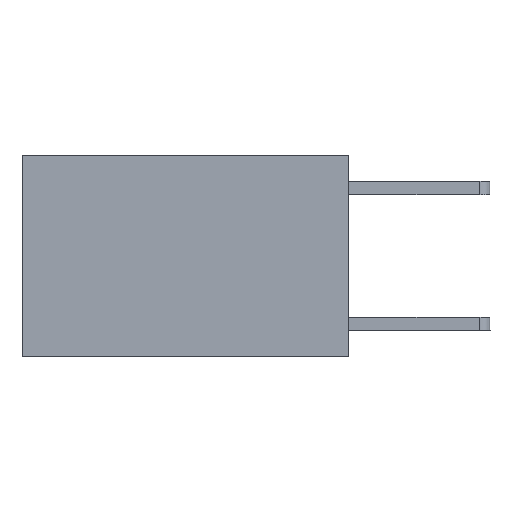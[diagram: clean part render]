
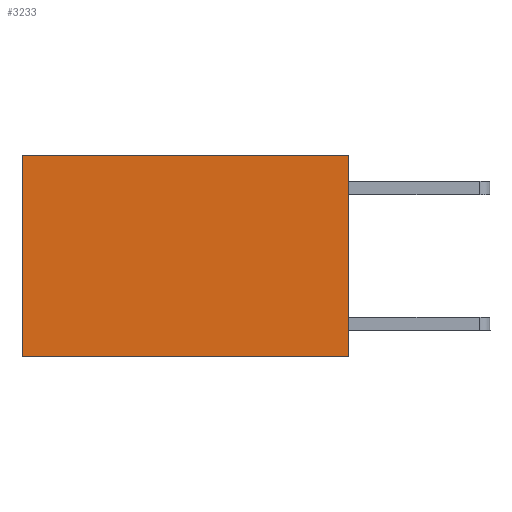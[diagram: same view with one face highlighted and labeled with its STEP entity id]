
A CAD part, left-side view. The second image highlights one B-rep face of the part: STEP entity #3233.
In plain terms, the highlighted planar face has unit normal (-1, 0, 0).
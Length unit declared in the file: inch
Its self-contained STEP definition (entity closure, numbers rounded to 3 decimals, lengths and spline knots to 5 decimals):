
#50 = EDGE_LOOP ( 'NONE', ( #3849, #9627, #2317, #8658 ) ) ;
#349 = EDGE_CURVE ( 'NONE', #6914, #4765, #1908, .T. ) ;
#634 = EDGE_CURVE ( 'NONE', #9391, #4765, #9523, .T. ) ;
#692 = EDGE_CURVE ( 'NONE', #8015, #9391, #9375, .T. ) ;
#1427 = CARTESIAN_POINT ( 'NONE',  ( 0.2625, 0.6, 0. ) ) ;
#1551 = DIRECTION ( 'NONE',  ( 0., 0., -1. ) ) ;
#1572 = CARTESIAN_POINT ( 'NONE',  ( 0.2625, 0.6, -0.37 ) ) ;
#1664 = VECTOR ( 'NONE', #1551, 39.37008 ) ;
#1908 = LINE ( 'NONE', #1427, #1664 ) ;
#2317 = ORIENTED_EDGE ( 'NONE', *, *, #692, .F. ) ;
#2415 = AXIS2_PLACEMENT_3D ( 'NONE', #9315, #6170, #7320 ) ;
#3233 = ADVANCED_FACE ( 'NONE', ( #3497 ), #9652, .F. ) ;
#3382 = CARTESIAN_POINT ( 'NONE',  ( 0.2625, 0., 0. ) ) ;
#3497 = FACE_OUTER_BOUND ( 'NONE', #50, .T. ) ;
#3748 = DIRECTION ( 'NONE',  ( 0., 0., -1. ) ) ;
#3849 = ORIENTED_EDGE ( 'NONE', *, *, #349, .T. ) ;
#4765 = VERTEX_POINT ( 'NONE', #1572 ) ;
#4825 = EDGE_CURVE ( 'NONE', #8015, #6914, #9385, .T. ) ;
#5110 = CARTESIAN_POINT ( 'NONE',  ( 0.2625, 0., 0. ) ) ;
#5521 = CARTESIAN_POINT ( 'NONE',  ( 0.2625, 0., -0.37 ) ) ;
#5523 = DIRECTION ( 'NONE',  ( 0., 1., 0. ) ) ;
#6170 = DIRECTION ( 'NONE',  ( 1., 0., 0. ) ) ;
#6895 = CARTESIAN_POINT ( 'NONE',  ( 0.2625, 0., -0.37 ) ) ;
#6914 = VERTEX_POINT ( 'NONE', #9634 ) ;
#7288 = CARTESIAN_POINT ( 'NONE',  ( 0.2625, 0., 0. ) ) ;
#7320 = DIRECTION ( 'NONE',  ( 0., 0., -1. ) ) ;
#7909 = VECTOR ( 'NONE', #8027, 39.37008 ) ;
#8015 = VERTEX_POINT ( 'NONE', #7288 ) ;
#8027 = DIRECTION ( 'NONE',  ( 0., 1., 0. ) ) ;
#8658 = ORIENTED_EDGE ( 'NONE', *, *, #4825, .T. ) ;
#9264 = VECTOR ( 'NONE', #3748, 39.37008 ) ;
#9315 = CARTESIAN_POINT ( 'NONE',  ( 0.2625, 0., 0. ) ) ;
#9375 = LINE ( 'NONE', #3382, #9264 ) ;
#9385 = LINE ( 'NONE', #5110, #7909 ) ;
#9391 = VERTEX_POINT ( 'NONE', #6895 ) ;
#9465 = VECTOR ( 'NONE', #5523, 39.37008 ) ;
#9523 = LINE ( 'NONE', #5521, #9465 ) ;
#9627 = ORIENTED_EDGE ( 'NONE', *, *, #634, .F. ) ;
#9634 = CARTESIAN_POINT ( 'NONE',  ( 0.2625, 0.6, 0. ) ) ;
#9652 = PLANE ( 'NONE',  #2415 ) ;
